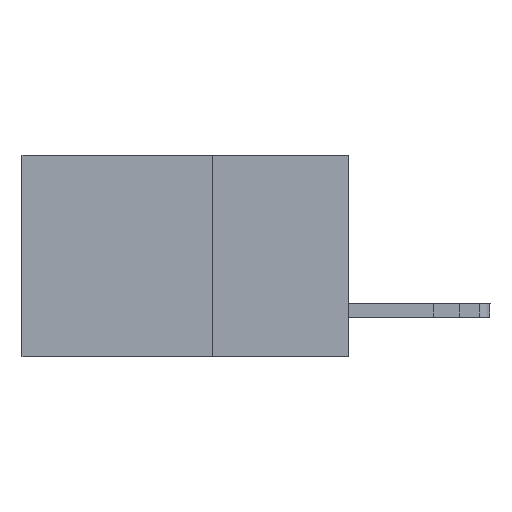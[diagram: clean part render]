
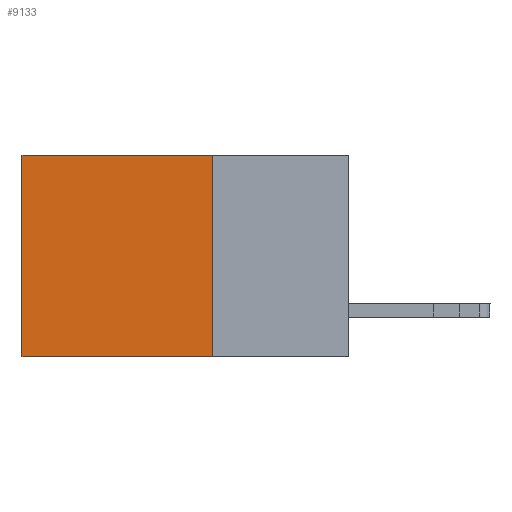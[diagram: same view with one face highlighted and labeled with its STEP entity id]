
A CAD part, left-side view. The second image highlights one B-rep face of the part: STEP entity #9133.
In plain terms, the highlighted planar face has unit normal (-1, 0, 0).
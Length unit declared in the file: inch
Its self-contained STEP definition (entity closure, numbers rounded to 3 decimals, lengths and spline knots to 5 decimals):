
#251 = EDGE_LOOP ( 'NONE', ( #14151, #2145, #14283, #13499 ) ) ;
#504 = DIRECTION ( 'NONE',  ( 0., 1., 0. ) ) ;
#693 = PLANE ( 'NONE',  #13850 ) ;
#922 = VECTOR ( 'NONE', #14358, 39.37008 ) ;
#1122 = LINE ( 'NONE', #6872, #8949 ) ;
#2145 = ORIENTED_EDGE ( 'NONE', *, *, #5094, .F. ) ;
#3080 = EDGE_CURVE ( 'NONE', #7479, #6752, #3356, .T. ) ;
#3346 = DIRECTION ( 'NONE',  ( 0., 0., -1. ) ) ;
#3356 = LINE ( 'NONE', #8500, #9927 ) ;
#4472 = CARTESIAN_POINT ( 'NONE',  ( 0.298, 0.25, -0.37 ) ) ;
#5094 = EDGE_CURVE ( 'NONE', #7436, #6752, #9190, .T. ) ;
#5176 = CARTESIAN_POINT ( 'NONE',  ( 0.298, 0.25, 0. ) ) ;
#5191 = CARTESIAN_POINT ( 'NONE',  ( 0.298, 0.6, -0.37 ) ) ;
#6173 = FACE_OUTER_BOUND ( 'NONE', #251, .T. ) ;
#6752 = VERTEX_POINT ( 'NONE', #5191 ) ;
#6872 = CARTESIAN_POINT ( 'NONE',  ( 0.298, 0.25, 0. ) ) ;
#7142 = DIRECTION ( 'NONE',  ( 0., 1., 0. ) ) ;
#7436 = VERTEX_POINT ( 'NONE', #4472 ) ;
#7479 = VERTEX_POINT ( 'NONE', #15796 ) ;
#7948 = LINE ( 'NONE', #5176, #922 ) ;
#8500 = CARTESIAN_POINT ( 'NONE',  ( 0.298, 0.6, 0. ) ) ;
#8949 = VECTOR ( 'NONE', #504, 39.37008 ) ;
#9133 = ADVANCED_FACE ( 'NONE', ( #6173 ), #693, .F. ) ;
#9190 = LINE ( 'NONE', #11554, #14734 ) ;
#9651 = DIRECTION ( 'NONE',  ( 0., 0., -1. ) ) ;
#9891 = CARTESIAN_POINT ( 'NONE',  ( 0.298, 0.25, 0. ) ) ;
#9927 = VECTOR ( 'NONE', #9651, 39.37008 ) ;
#10962 = CARTESIAN_POINT ( 'NONE',  ( 0.298, 0.25, 0. ) ) ;
#11203 = DIRECTION ( 'NONE',  ( 1., 0., 0. ) ) ;
#11380 = VERTEX_POINT ( 'NONE', #10962 ) ;
#11554 = CARTESIAN_POINT ( 'NONE',  ( 0.298, 0.25, -0.37 ) ) ;
#13499 = ORIENTED_EDGE ( 'NONE', *, *, #14876, .T. ) ;
#13850 = AXIS2_PLACEMENT_3D ( 'NONE', #9891, #11203, #3346 ) ;
#14151 = ORIENTED_EDGE ( 'NONE', *, *, #3080, .T. ) ;
#14283 = ORIENTED_EDGE ( 'NONE', *, *, #14456, .F. ) ;
#14358 = DIRECTION ( 'NONE',  ( 0., 0., -1. ) ) ;
#14456 = EDGE_CURVE ( 'NONE', #11380, #7436, #7948, .T. ) ;
#14734 = VECTOR ( 'NONE', #7142, 39.37008 ) ;
#14876 = EDGE_CURVE ( 'NONE', #11380, #7479, #1122, .T. ) ;
#15796 = CARTESIAN_POINT ( 'NONE',  ( 0.298, 0.6, 0. ) ) ;
